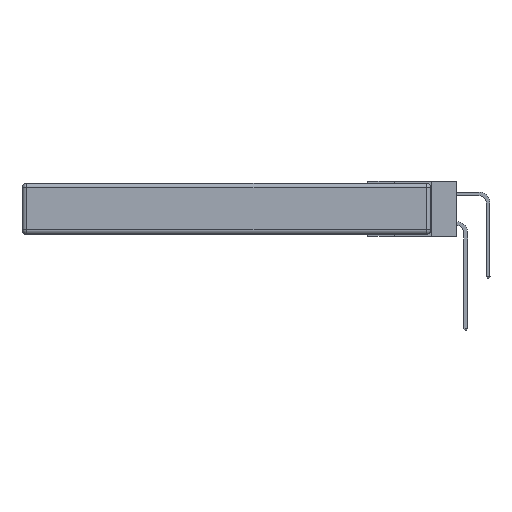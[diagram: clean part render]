
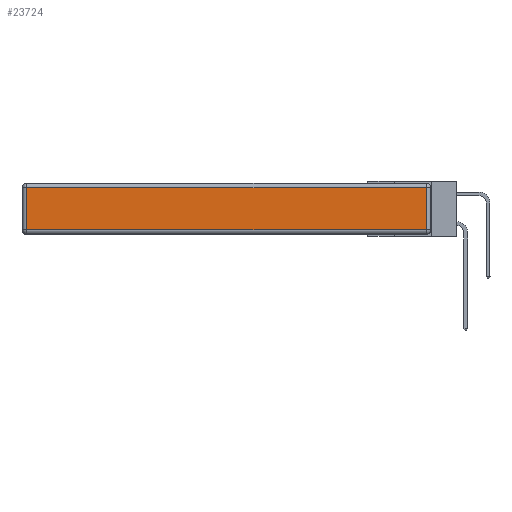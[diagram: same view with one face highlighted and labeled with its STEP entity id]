
A CAD part, left-side view. The second image highlights one B-rep face of the part: STEP entity #23724.
In plain terms, the highlighted planar face has unit normal (-1, 0, 0).
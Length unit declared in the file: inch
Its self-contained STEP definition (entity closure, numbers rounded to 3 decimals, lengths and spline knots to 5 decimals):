
#636 = CARTESIAN_POINT ( 'NONE',  ( 0., 2.72, -0.343 ) ) ;
#991 = LINE ( 'NONE', #4673, #8581 ) ;
#2472 = DIRECTION ( 'NONE',  ( 0., 0., 1. ) ) ;
#3023 = EDGE_LOOP ( 'NONE', ( #11779, #22453, #20627, #8721 ) ) ;
#3686 = VERTEX_POINT ( 'NONE', #3763 ) ;
#3763 = CARTESIAN_POINT ( 'NONE',  ( 0., 2.72, -0.313 ) ) ;
#4030 = VECTOR ( 'NONE', #4656, 39.37008 ) ;
#4048 = VERTEX_POINT ( 'NONE', #23374 ) ;
#4351 = LINE ( 'NONE', #18252, #23757 ) ;
#4656 = DIRECTION ( 'NONE',  ( 0., 0., 1. ) ) ;
#4673 = CARTESIAN_POINT ( 'NONE',  ( 0., 2.75, -0.03 ) ) ;
#4931 = VECTOR ( 'NONE', #15047, 39.37008 ) ;
#6447 = DIRECTION ( 'NONE',  ( 0., 1., 0. ) ) ;
#6524 = CARTESIAN_POINT ( 'NONE',  ( 0., 0.03, -0.343 ) ) ;
#8022 = DIRECTION ( 'NONE',  ( 0., -1., 0. ) ) ;
#8072 = CARTESIAN_POINT ( 'NONE',  ( 0., 0.03, -0.313 ) ) ;
#8172 = LINE ( 'NONE', #6524, #4030 ) ;
#8581 = VECTOR ( 'NONE', #6447, 39.37008 ) ;
#8721 = ORIENTED_EDGE ( 'NONE', *, *, #12031, .T. ) ;
#10961 = EDGE_CURVE ( 'NONE', #3686, #12596, #4351, .T. ) ;
#11779 = ORIENTED_EDGE ( 'NONE', *, *, #10961, .T. ) ;
#12031 = EDGE_CURVE ( 'NONE', #23015, #3686, #12597, .T. ) ;
#12596 = VERTEX_POINT ( 'NONE', #8072 ) ;
#12597 = LINE ( 'NONE', #636, #4931 ) ;
#12636 = CARTESIAN_POINT ( 'NONE',  ( 0., 2.72, -0.03 ) ) ;
#15047 = DIRECTION ( 'NONE',  ( 0., 0., -1. ) ) ;
#15994 = EDGE_CURVE ( 'NONE', #4048, #23015, #991, .T. ) ;
#16476 = DIRECTION ( 'NONE',  ( -1., 0., 0. ) ) ;
#18252 = CARTESIAN_POINT ( 'NONE',  ( 0., 0., -0.313 ) ) ;
#18632 = CARTESIAN_POINT ( 'NONE',  ( 0., 0., -0.343 ) ) ;
#20627 = ORIENTED_EDGE ( 'NONE', *, *, #15994, .T. ) ;
#20767 = PLANE ( 'NONE',  #23557 ) ;
#22453 = ORIENTED_EDGE ( 'NONE', *, *, #23798, .T. ) ;
#23015 = VERTEX_POINT ( 'NONE', #12636 ) ;
#23374 = CARTESIAN_POINT ( 'NONE',  ( 0., 0.03, -0.03 ) ) ;
#23557 = AXIS2_PLACEMENT_3D ( 'NONE', #18632, #16476, #2472 ) ;
#23724 = ADVANCED_FACE ( 'NONE', ( #25977 ), #20767, .T. ) ;
#23757 = VECTOR ( 'NONE', #8022, 39.37008 ) ;
#23798 = EDGE_CURVE ( 'NONE', #12596, #4048, #8172, .T. ) ;
#25977 = FACE_OUTER_BOUND ( 'NONE', #3023, .T. ) ;
